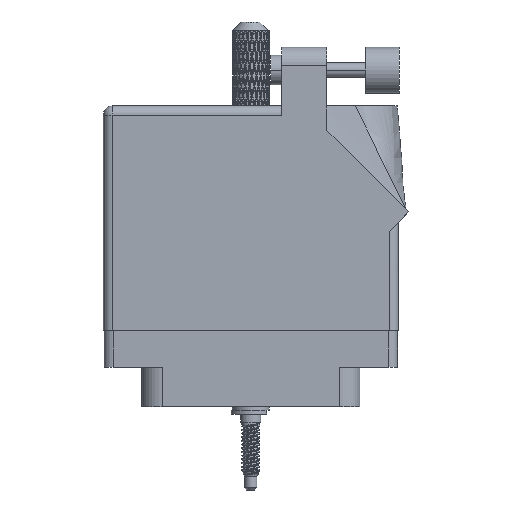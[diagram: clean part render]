
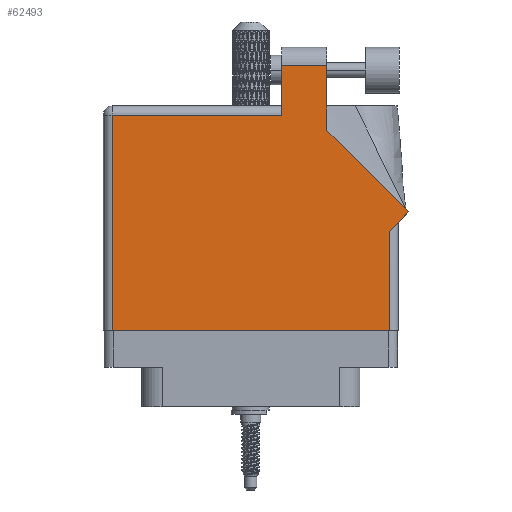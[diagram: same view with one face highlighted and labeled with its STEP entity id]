
A CAD part, front view. The second image highlights one B-rep face of the part: STEP entity #62493.
In plain terms, the highlighted face is planar.
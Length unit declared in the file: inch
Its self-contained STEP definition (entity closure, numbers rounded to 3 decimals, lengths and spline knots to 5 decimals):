
#1242 = CARTESIAN_POINT ( 'NONE',  ( -1.005, 1.368, 0.455 ) ) ;
#4382 = VECTOR ( 'NONE', #53531, 39.37008 ) ;
#4481 = FACE_OUTER_BOUND ( 'NONE', #74947, .T. ) ;
#7075 = VECTOR ( 'NONE', #25867, 39.37008 ) ;
#7247 = CARTESIAN_POINT ( 'NONE',  ( 0.519, 1.26442, 0.455 ) ) ;
#10490 = LINE ( 'NONE', #33582, #90384 ) ;
#11808 = DIRECTION ( 'NONE',  ( 0., -1., 0. ) ) ;
#13214 = EDGE_CURVE ( 'NONE', #22148, #98872, #46806, .T. ) ;
#14082 = DIRECTION ( 'NONE',  ( 0., 0., -1. ) ) ;
#15567 = CARTESIAN_POINT ( 'NONE',  ( 0.519, 1.705, 0.455 ) ) ;
#18337 = CARTESIAN_POINT ( 'NONE',  ( 1.07571, 0.70771, 0.455 ) ) ;
#18656 = ORIENTED_EDGE ( 'NONE', *, *, #13214, .T. ) ;
#20489 = ORIENTED_EDGE ( 'NONE', *, *, #74917, .T. ) ;
#22148 = VERTEX_POINT ( 'NONE', #7247 ) ;
#23138 = LINE ( 'NONE', #88482, #53165 ) ;
#23601 = VERTEX_POINT ( 'NONE', #74118 ) ;
#25867 = DIRECTION ( 'NONE',  ( -1., 0., 0. ) ) ;
#27363 = CARTESIAN_POINT ( 'NONE',  ( -0.943, -0.1, 0.455 ) ) ;
#28851 = CARTESIAN_POINT ( 'NONE',  ( 1.005, 0.637, 0.455 ) ) ;
#33582 = CARTESIAN_POINT ( 'NONE',  ( 0.943, 0.637, 0.455 ) ) ;
#34375 = LINE ( 'NONE', #27363, #49391 ) ;
#35180 = VECTOR ( 'NONE', #78911, 39.37008 ) ;
#36119 = AXIS2_PLACEMENT_3D ( 'NONE', #103535, #14082, #46804 ) ;
#37181 = PLANE ( 'NONE',  #36119 ) ;
#37367 = EDGE_CURVE ( 'NONE', #98872, #71471, #57383, .T. ) ;
#39781 = EDGE_CURVE ( 'NONE', #97519, #51172, #10490, .T. ) ;
#40566 = CARTESIAN_POINT ( 'NONE',  ( 0.212, 1.705, 0.455 ) ) ;
#40838 = EDGE_CURVE ( 'NONE', #51172, #23601, #52999, .T. ) ;
#42126 = ORIENTED_EDGE ( 'NONE', *, *, #57868, .T. ) ;
#44236 = ORIENTED_EDGE ( 'NONE', *, *, #40838, .T. ) ;
#46282 = CARTESIAN_POINT ( 'NONE',  ( 0.519, 1.26442, 0.455 ) ) ;
#46804 = DIRECTION ( 'NONE',  ( -1., 0., 0. ) ) ;
#46806 = LINE ( 'NONE', #46282, #35180 ) ;
#47767 = ORIENTED_EDGE ( 'NONE', *, *, #90286, .T. ) ;
#48214 = CARTESIAN_POINT ( 'NONE',  ( -0.943, -0.1, 0.455 ) ) ;
#48998 = ORIENTED_EDGE ( 'NONE', *, *, #98541, .T. ) ;
#49161 = DIRECTION ( 'NONE',  ( 0., 1., 0. ) ) ;
#49391 = VECTOR ( 'NONE', #58465, 39.37008 ) ;
#50129 = VERTEX_POINT ( 'NONE', #80571 ) ;
#50976 = DIRECTION ( 'NONE',  ( 1., 0., 0. ) ) ;
#51087 = DIRECTION ( 'NONE',  ( -0.707, 0.707, 0. ) ) ;
#51172 = VERTEX_POINT ( 'NONE', #88086 ) ;
#52999 = LINE ( 'NONE', #28851, #4382 ) ;
#53165 = VECTOR ( 'NONE', #50976, 39.37008 ) ;
#53531 = DIRECTION ( 'NONE',  ( 0.707, 0.707, 0. ) ) ;
#54358 = VECTOR ( 'NONE', #99650, 39.37008 ) ;
#57383 = LINE ( 'NONE', #80948, #54358 ) ;
#57868 = EDGE_CURVE ( 'NONE', #71471, #74575, #90730, .T. ) ;
#58465 = DIRECTION ( 'NONE',  ( 0., -1., 0. ) ) ;
#60241 = ORIENTED_EDGE ( 'NONE', *, *, #37367, .T. ) ;
#62105 = ORIENTED_EDGE ( 'NONE', *, *, #78575, .T. ) ;
#62493 = ADVANCED_FACE ( 'NONE', ( #4481 ), #37181, .F. ) ;
#71471 = VERTEX_POINT ( 'NONE', #40566 ) ;
#73376 = VECTOR ( 'NONE', #11808, 39.37008 ) ;
#74118 = CARTESIAN_POINT ( 'NONE',  ( 1.07571, 0.70771, 0.455 ) ) ;
#74575 = VERTEX_POINT ( 'NONE', #90824 ) ;
#74917 = EDGE_CURVE ( 'NONE', #23601, #22148, #100311, .T. ) ;
#74947 = EDGE_LOOP ( 'NONE', ( #18656, #60241, #42126, #48998, #62105, #47767, #86097, #44236, #20489 ) ) ;
#78575 = EDGE_CURVE ( 'NONE', #50129, #97591, #34375, .T. ) ;
#78911 = DIRECTION ( 'NONE',  ( 0., 1., 0. ) ) ;
#80571 = CARTESIAN_POINT ( 'NONE',  ( -0.943, 1.368, 0.455 ) ) ;
#80948 = CARTESIAN_POINT ( 'NONE',  ( 0.212, 1.705, 0.455 ) ) ;
#82136 = LINE ( 'NONE', #1242, #7075 ) ;
#85196 = CARTESIAN_POINT ( 'NONE',  ( 0.212, 1.43, 0.455 ) ) ;
#86097 = ORIENTED_EDGE ( 'NONE', *, *, #39781, .T. ) ;
#88086 = CARTESIAN_POINT ( 'NONE',  ( 0.943, 0.575, 0.455 ) ) ;
#88482 = CARTESIAN_POINT ( 'NONE',  ( -1.005, -0.1, 0.455 ) ) ;
#90286 = EDGE_CURVE ( 'NONE', #97591, #97519, #23138, .T. ) ;
#90384 = VECTOR ( 'NONE', #49161, 39.37008 ) ;
#90730 = LINE ( 'NONE', #85196, #73376 ) ;
#90824 = CARTESIAN_POINT ( 'NONE',  ( 0.212, 1.368, 0.455 ) ) ;
#93932 = VECTOR ( 'NONE', #51087, 39.37008 ) ;
#97519 = VERTEX_POINT ( 'NONE', #101758 ) ;
#97591 = VERTEX_POINT ( 'NONE', #48214 ) ;
#98541 = EDGE_CURVE ( 'NONE', #74575, #50129, #82136, .T. ) ;
#98872 = VERTEX_POINT ( 'NONE', #15567 ) ;
#99650 = DIRECTION ( 'NONE',  ( -1., 0., 0. ) ) ;
#100311 = LINE ( 'NONE', #18337, #93932 ) ;
#101758 = CARTESIAN_POINT ( 'NONE',  ( 0.943, -0.1, 0.455 ) ) ;
#103535 = CARTESIAN_POINT ( 'NONE',  ( -1.005, 1.43, 0.455 ) ) ;
